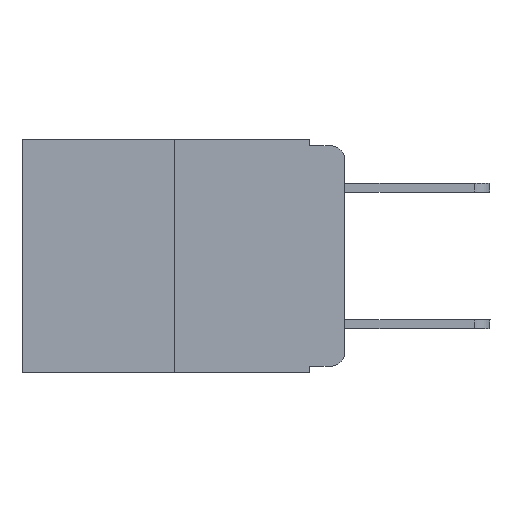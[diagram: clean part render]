
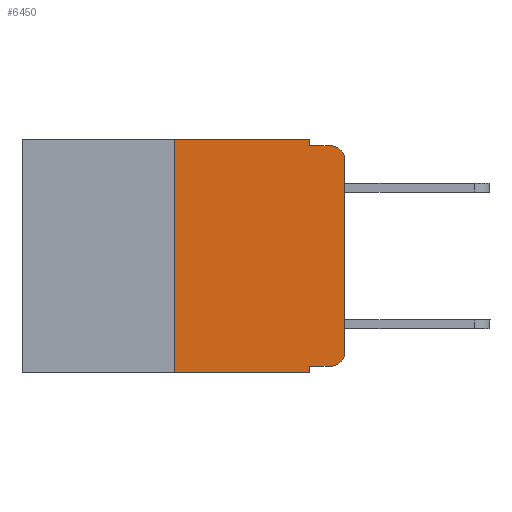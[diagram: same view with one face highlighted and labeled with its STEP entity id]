
A CAD part, left-side view. The second image highlights one B-rep face of the part: STEP entity #6450.
In plain terms, the highlighted planar face has unit normal (-1, 0, 0).
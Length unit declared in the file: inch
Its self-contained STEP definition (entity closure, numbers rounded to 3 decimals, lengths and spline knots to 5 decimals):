
#14 = CARTESIAN_POINT ( 'NONE',  ( 0., 0.25, 0. ) ) ;
#86 = DIRECTION ( 'NONE',  ( 0., -1., 0. ) ) ;
#190 = LINE ( 'NONE', #8731, #881 ) ;
#297 = LINE ( 'NONE', #4820, #12491 ) ;
#601 = DIRECTION ( 'NONE',  ( 0., 0., -1. ) ) ;
#694 = CARTESIAN_POINT ( 'NONE',  ( 0., 0.051, 0. ) ) ;
#707 = EDGE_CURVE ( 'NONE', #13651, #902, #5639, .T. ) ;
#735 = CARTESIAN_POINT ( 'NONE',  ( 0., 0.02, -0.01 ) ) ;
#881 = VECTOR ( 'NONE', #9866, 39.37008 ) ;
#902 = VERTEX_POINT ( 'NONE', #9990 ) ;
#1021 = LINE ( 'NONE', #694, #3104 ) ;
#1606 = CARTESIAN_POINT ( 'NONE',  ( 0., 0.051, 0. ) ) ;
#1740 = VERTEX_POINT ( 'NONE', #8779 ) ;
#1748 = EDGE_CURVE ( 'NONE', #1740, #10388, #190, .T. ) ;
#2759 = ORIENTED_EDGE ( 'NONE', *, *, #4320, .F. ) ;
#2923 = VECTOR ( 'NONE', #10805, 39.37008 ) ;
#2976 = CARTESIAN_POINT ( 'NONE',  ( 0., 0.473, 0. ) ) ;
#2981 = DIRECTION ( 'NONE',  ( -1., 0., 0. ) ) ;
#3104 = VECTOR ( 'NONE', #11425, 39.37008 ) ;
#3191 = VECTOR ( 'NONE', #601, 39.37008 ) ;
#3485 = CARTESIAN_POINT ( 'NONE',  ( 0., 0.051, -0.01 ) ) ;
#3795 = DIRECTION ( 'NONE',  ( 0., -1., 0. ) ) ;
#3823 = AXIS2_PLACEMENT_3D ( 'NONE', #2976, #6362, #4211 ) ;
#3824 = CARTESIAN_POINT ( 'NONE',  ( 0., 0.051, 0. ) ) ;
#3963 = CARTESIAN_POINT ( 'NONE',  ( 0., 0.02, -0.03 ) ) ;
#4008 = DIRECTION ( 'NONE',  ( 0., 0., -1. ) ) ;
#4211 = DIRECTION ( 'NONE',  ( 0., 0., -1. ) ) ;
#4215 = CARTESIAN_POINT ( 'NONE',  ( 0., 0.02, -0.313 ) ) ;
#4320 = EDGE_CURVE ( 'NONE', #11763, #5854, #1021, .T. ) ;
#4362 = VERTEX_POINT ( 'NONE', #735 ) ;
#4820 = CARTESIAN_POINT ( 'NONE',  ( 0., 0.051, -0.01 ) ) ;
#4865 = ORIENTED_EDGE ( 'NONE', *, *, #1748, .T. ) ;
#4954 = DIRECTION ( 'NONE',  ( -1., 0., 0. ) ) ;
#5639 = LINE ( 'NONE', #10452, #7172 ) ;
#5756 = CARTESIAN_POINT ( 'NONE',  ( 0., 0., -0.03 ) ) ;
#5854 = VERTEX_POINT ( 'NONE', #3485 ) ;
#6313 = PLANE ( 'NONE',  #3823 ) ;
#6362 = DIRECTION ( 'NONE',  ( 1., 0., 0. ) ) ;
#6450 = ADVANCED_FACE ( 'NONE', ( #7927 ), #6313, .F. ) ;
#7172 = VECTOR ( 'NONE', #3795, 39.37008 ) ;
#7191 = EDGE_LOOP ( 'NONE', ( #4865, #12032, #8155, #2759, #7735, #13496, #10241, #11935, #11664, #10736 ) ) ;
#7733 = CIRCLE ( 'NONE', #11810, 0.02 ) ;
#7735 = ORIENTED_EDGE ( 'NONE', *, *, #9086, .F. ) ;
#7842 = EDGE_CURVE ( 'NONE', #12805, #13098, #12146, .T. ) ;
#7927 = FACE_OUTER_BOUND ( 'NONE', #7191, .T. ) ;
#8155 = ORIENTED_EDGE ( 'NONE', *, *, #10317, .F. ) ;
#8199 = EDGE_CURVE ( 'NONE', #902, #1740, #7733, .T. ) ;
#8345 = CIRCLE ( 'NONE', #12187, 0.02 ) ;
#8403 = VECTOR ( 'NONE', #86, 39.37008 ) ;
#8731 = CARTESIAN_POINT ( 'NONE',  ( 0., 0., 0. ) ) ;
#8779 = CARTESIAN_POINT ( 'NONE',  ( 0., 0., -0.313 ) ) ;
#9086 = EDGE_CURVE ( 'NONE', #12736, #11763, #11431, .T. ) ;
#9495 = DIRECTION ( 'NONE',  ( 0., 0., -1. ) ) ;
#9793 = CARTESIAN_POINT ( 'NONE',  ( 0., 0.473, -0.343 ) ) ;
#9866 = DIRECTION ( 'NONE',  ( 0., 0., 1. ) ) ;
#9990 = CARTESIAN_POINT ( 'NONE',  ( 0., 0.02, -0.333 ) ) ;
#10055 = CARTESIAN_POINT ( 'NONE',  ( 0., 0.051, -0.333 ) ) ;
#10241 = ORIENTED_EDGE ( 'NONE', *, *, #7842, .T. ) ;
#10317 = EDGE_CURVE ( 'NONE', #5854, #4362, #297, .T. ) ;
#10388 = VERTEX_POINT ( 'NONE', #5756 ) ;
#10452 = CARTESIAN_POINT ( 'NONE',  ( 0., 0.051, -0.333 ) ) ;
#10488 = EDGE_CURVE ( 'NONE', #13651, #13098, #11983, .T. ) ;
#10736 = ORIENTED_EDGE ( 'NONE', *, *, #8199, .T. ) ;
#10805 = DIRECTION ( 'NONE',  ( 0., 0., 1. ) ) ;
#11259 = DIRECTION ( 'NONE',  ( 0., -1., 0. ) ) ;
#11265 = VECTOR ( 'NONE', #11259, 39.37008 ) ;
#11380 = CARTESIAN_POINT ( 'NONE',  ( 0., 0.051, -0.343 ) ) ;
#11425 = DIRECTION ( 'NONE',  ( 0., 0., -1. ) ) ;
#11431 = LINE ( 'NONE', #12273, #11265 ) ;
#11664 = ORIENTED_EDGE ( 'NONE', *, *, #707, .T. ) ;
#11732 = CARTESIAN_POINT ( 'NONE',  ( 0., 0.25, 0. ) ) ;
#11763 = VERTEX_POINT ( 'NONE', #1606 ) ;
#11810 = AXIS2_PLACEMENT_3D ( 'NONE', #4215, #2981, #9495 ) ;
#11862 = CARTESIAN_POINT ( 'NONE',  ( 0., 0.25, -0.343 ) ) ;
#11908 = EDGE_CURVE ( 'NONE', #10388, #4362, #8345, .T. ) ;
#11935 = ORIENTED_EDGE ( 'NONE', *, *, #10488, .F. ) ;
#11983 = LINE ( 'NONE', #3824, #3191 ) ;
#12032 = ORIENTED_EDGE ( 'NONE', *, *, #11908, .T. ) ;
#12146 = LINE ( 'NONE', #9793, #8403 ) ;
#12187 = AXIS2_PLACEMENT_3D ( 'NONE', #3963, #4954, #4008 ) ;
#12273 = CARTESIAN_POINT ( 'NONE',  ( 0., 0.473, 0. ) ) ;
#12371 = DIRECTION ( 'NONE',  ( 0., -1., 0. ) ) ;
#12491 = VECTOR ( 'NONE', #12371, 39.37008 ) ;
#12736 = VERTEX_POINT ( 'NONE', #11732 ) ;
#12805 = VERTEX_POINT ( 'NONE', #11862 ) ;
#13098 = VERTEX_POINT ( 'NONE', #11380 ) ;
#13220 = LINE ( 'NONE', #14, #2923 ) ;
#13410 = EDGE_CURVE ( 'NONE', #12805, #12736, #13220, .T. ) ;
#13496 = ORIENTED_EDGE ( 'NONE', *, *, #13410, .F. ) ;
#13651 = VERTEX_POINT ( 'NONE', #10055 ) ;
